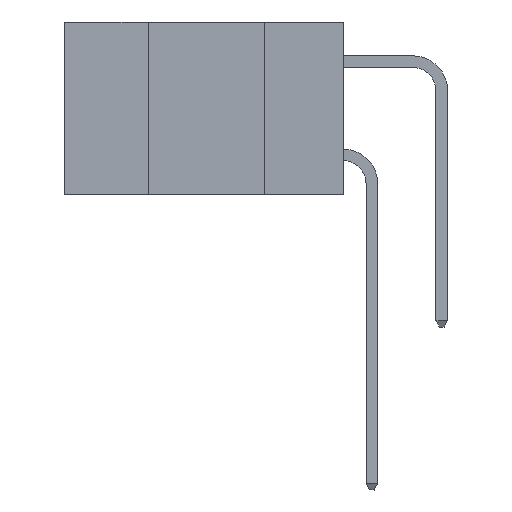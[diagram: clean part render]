
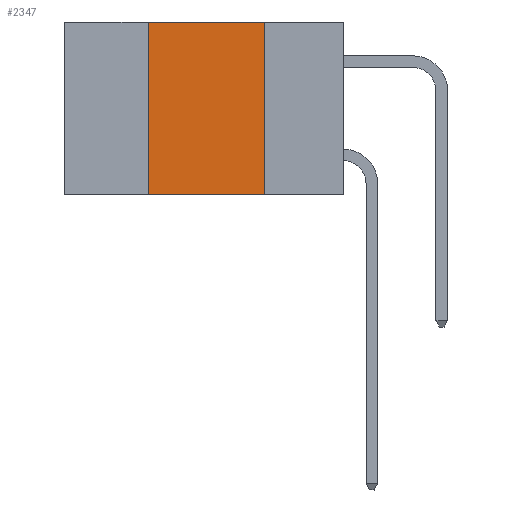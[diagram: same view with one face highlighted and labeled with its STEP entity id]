
A CAD part, left-side view. The second image highlights one B-rep face of the part: STEP entity #2347.
In plain terms, the highlighted planar face has unit normal (-1, 0, 0).
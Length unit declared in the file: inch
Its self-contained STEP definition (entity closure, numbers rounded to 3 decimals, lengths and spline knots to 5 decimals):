
#192 = EDGE_CURVE ( 'NONE', #541, #11665, #1806, .T. ) ;
#332 = CARTESIAN_POINT ( 'NONE',  ( 0., 0.42, -0.37 ) ) ;
#541 = VERTEX_POINT ( 'NONE', #17014 ) ;
#566 = ORIENTED_EDGE ( 'NONE', *, *, #17976, .T. ) ;
#945 = VERTEX_POINT ( 'NONE', #3938 ) ;
#1332 = LINE ( 'NONE', #11568, #7219 ) ;
#1577 = DIRECTION ( 'NONE',  ( 1., 0., 0. ) ) ;
#1806 = LINE ( 'NONE', #332, #16730 ) ;
#2184 = ORIENTED_EDGE ( 'NONE', *, *, #5947, .F. ) ;
#2347 = ADVANCED_FACE ( 'NONE', ( #9316 ), #7923, .F. ) ;
#2673 = LINE ( 'NONE', #5559, #12036 ) ;
#2820 = AXIS2_PLACEMENT_3D ( 'NONE', #5680, #1577, #9852 ) ;
#2930 = DIRECTION ( 'NONE',  ( 0., -1., 0. ) ) ;
#3797 = VECTOR ( 'NONE', #9796, 39.37008 ) ;
#3938 = CARTESIAN_POINT ( 'NONE',  ( 0., 0.17, 0. ) ) ;
#4714 = DIRECTION ( 'NONE',  ( 0., 0., 1. ) ) ;
#5559 = CARTESIAN_POINT ( 'NONE',  ( 0., 0.17, -0.37 ) ) ;
#5680 = CARTESIAN_POINT ( 'NONE',  ( 0., 0.6, 0. ) ) ;
#5947 = EDGE_CURVE ( 'NONE', #11665, #945, #1332, .T. ) ;
#7219 = VECTOR ( 'NONE', #2930, 39.37008 ) ;
#7419 = ORIENTED_EDGE ( 'NONE', *, *, #192, .F. ) ;
#7923 = PLANE ( 'NONE',  #2820 ) ;
#8306 = LINE ( 'NONE', #11212, #3797 ) ;
#8699 = ORIENTED_EDGE ( 'NONE', *, *, #16289, .F. ) ;
#9316 = FACE_OUTER_BOUND ( 'NONE', #13099, .T. ) ;
#9796 = DIRECTION ( 'NONE',  ( 0., -1., 0. ) ) ;
#9814 = DIRECTION ( 'NONE',  ( 0., 0., -1. ) ) ;
#9852 = DIRECTION ( 'NONE',  ( 0., 0., -1. ) ) ;
#11212 = CARTESIAN_POINT ( 'NONE',  ( 0., 0.6, -0.37 ) ) ;
#11568 = CARTESIAN_POINT ( 'NONE',  ( 0., 0.6, 0. ) ) ;
#11665 = VERTEX_POINT ( 'NONE', #15077 ) ;
#12036 = VECTOR ( 'NONE', #9814, 39.37008 ) ;
#13099 = EDGE_LOOP ( 'NONE', ( #8699, #2184, #7419, #566 ) ) ;
#15077 = CARTESIAN_POINT ( 'NONE',  ( 0., 0.42, 0. ) ) ;
#16220 = CARTESIAN_POINT ( 'NONE',  ( 0., 0.17, -0.37 ) ) ;
#16289 = EDGE_CURVE ( 'NONE', #945, #17647, #2673, .T. ) ;
#16730 = VECTOR ( 'NONE', #4714, 39.37008 ) ;
#17014 = CARTESIAN_POINT ( 'NONE',  ( 0., 0.42, -0.37 ) ) ;
#17647 = VERTEX_POINT ( 'NONE', #16220 ) ;
#17976 = EDGE_CURVE ( 'NONE', #541, #17647, #8306, .T. ) ;
